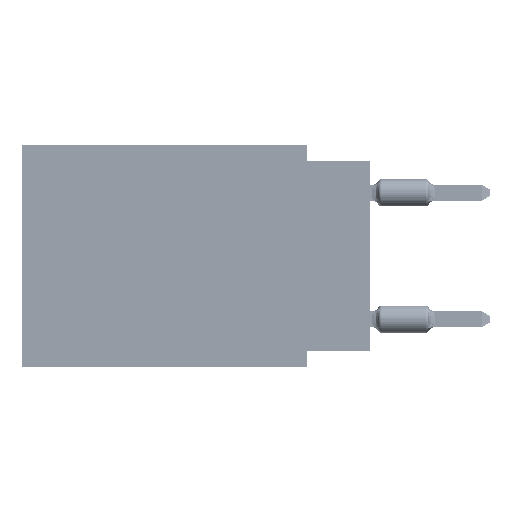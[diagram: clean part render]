
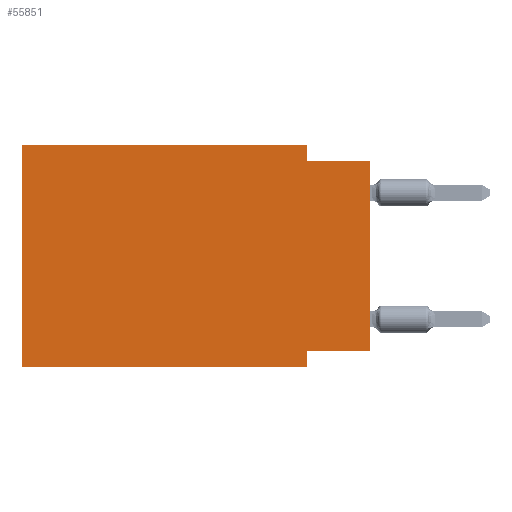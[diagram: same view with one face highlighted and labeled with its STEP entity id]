
A CAD part, left-side view. The second image highlights one B-rep face of the part: STEP entity #55851.
In plain terms, the highlighted planar face has unit normal (-1, 0, 0).
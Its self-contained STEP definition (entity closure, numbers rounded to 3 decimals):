
#151 = DIRECTION ( 'NONE',  ( 0., 0., 1. ) ) ;
#384 = CARTESIAN_POINT ( 'NONE',  ( 0., 2.54, -8.255 ) ) ;
#498 = LINE ( 'NONE', #28126, #64078 ) ;
#752 = LINE ( 'NONE', #40305, #62129 ) ;
#1316 = LINE ( 'NONE', #18832, #39171 ) ;
#3480 = EDGE_CURVE ( 'NONE', #56586, #4489, #69816, .T. ) ;
#4046 = FACE_OUTER_BOUND ( 'NONE', #61465, .T. ) ;
#4489 = VERTEX_POINT ( 'NONE', #43810 ) ;
#7274 = ORIENTED_EDGE ( 'NONE', *, *, #3480, .F. ) ;
#11560 = ORIENTED_EDGE ( 'NONE', *, *, #73206, .T. ) ;
#12030 = VERTEX_POINT ( 'NONE', #384 ) ;
#13238 = DIRECTION ( 'NONE',  ( 0., 0., 1. ) ) ;
#13810 = ORIENTED_EDGE ( 'NONE', *, *, #58039, .F. ) ;
#15136 = CARTESIAN_POINT ( 'NONE',  ( 0., 0., -0.635 ) ) ;
#16804 = VECTOR ( 'NONE', #53622, 1000. ) ;
#17238 = VERTEX_POINT ( 'NONE', #17566 ) ;
#17566 = CARTESIAN_POINT ( 'NONE',  ( 0., 2.54, -8.89 ) ) ;
#18680 = CARTESIAN_POINT ( 'NONE',  ( 0., 13.97, 0. ) ) ;
#18832 = CARTESIAN_POINT ( 'NONE',  ( 0., 0., 0. ) ) ;
#20469 = DIRECTION ( 'NONE',  ( 0., -1., 0. ) ) ;
#21967 = VECTOR ( 'NONE', #20469, 1000. ) ;
#23077 = DIRECTION ( 'NONE',  ( 0., 0., -1. ) ) ;
#25685 = CARTESIAN_POINT ( 'NONE',  ( 0., 13.97, -8.89 ) ) ;
#26681 = ORIENTED_EDGE ( 'NONE', *, *, #31737, .F. ) ;
#26885 = CARTESIAN_POINT ( 'NONE',  ( 0., 2.54, -0.635 ) ) ;
#28126 = CARTESIAN_POINT ( 'NONE',  ( 0., 0., -8.255 ) ) ;
#29567 = VECTOR ( 'NONE', #68330, 1000. ) ;
#31737 = EDGE_CURVE ( 'NONE', #34360, #44378, #38281, .T. ) ;
#34360 = VERTEX_POINT ( 'NONE', #26885 ) ;
#36318 = VERTEX_POINT ( 'NONE', #40016 ) ;
#38281 = LINE ( 'NONE', #67753, #40577 ) ;
#38374 = CARTESIAN_POINT ( 'NONE',  ( 0., 13.97, 0. ) ) ;
#39138 = ORIENTED_EDGE ( 'NONE', *, *, #44865, .F. ) ;
#39171 = VECTOR ( 'NONE', #13238, 1000. ) ;
#40016 = CARTESIAN_POINT ( 'NONE',  ( 0., 0., -8.255 ) ) ;
#40305 = CARTESIAN_POINT ( 'NONE',  ( 0., 2.54, -8.89 ) ) ;
#40577 = VECTOR ( 'NONE', #49110, 1000. ) ;
#40936 = LINE ( 'NONE', #41682, #16804 ) ;
#41682 = CARTESIAN_POINT ( 'NONE',  ( 0., 2.54, 0. ) ) ;
#43586 = AXIS2_PLACEMENT_3D ( 'NONE', #38374, #45809, #23077 ) ;
#43810 = CARTESIAN_POINT ( 'NONE',  ( 0., 2.54, 0. ) ) ;
#44072 = EDGE_CURVE ( 'NONE', #4489, #34360, #40936, .T. ) ;
#44378 = VERTEX_POINT ( 'NONE', #15136 ) ;
#44519 = LINE ( 'NONE', #67313, #54028 ) ;
#44865 = EDGE_CURVE ( 'NONE', #12030, #17238, #752, .T. ) ;
#45809 = DIRECTION ( 'NONE',  ( 1., 0., 0. ) ) ;
#46023 = ORIENTED_EDGE ( 'NONE', *, *, #49170, .T. ) ;
#46474 = CARTESIAN_POINT ( 'NONE',  ( 0., 13.97, -8.89 ) ) ;
#49031 = CARTESIAN_POINT ( 'NONE',  ( 0., 13.97, 0. ) ) ;
#49110 = DIRECTION ( 'NONE',  ( 0., -1., 0. ) ) ;
#49170 = EDGE_CURVE ( 'NONE', #56388, #17238, #60737, .T. ) ;
#53622 = DIRECTION ( 'NONE',  ( 0., 0., -1. ) ) ;
#54028 = VECTOR ( 'NONE', #151, 1000. ) ;
#55851 = ADVANCED_FACE ( 'NONE', ( #4046 ), #72357, .F. ) ;
#56388 = VERTEX_POINT ( 'NONE', #46474 ) ;
#56586 = VERTEX_POINT ( 'NONE', #49031 ) ;
#57839 = DIRECTION ( 'NONE',  ( 0., 0., -1. ) ) ;
#58039 = EDGE_CURVE ( 'NONE', #36318, #12030, #498, .T. ) ;
#60131 = ORIENTED_EDGE ( 'NONE', *, *, #44072, .F. ) ;
#60737 = LINE ( 'NONE', #25685, #21967 ) ;
#61465 = EDGE_LOOP ( 'NONE', ( #11560, #26681, #60131, #7274, #62051, #46023, #39138, #13810 ) ) ;
#62051 = ORIENTED_EDGE ( 'NONE', *, *, #68097, .F. ) ;
#62129 = VECTOR ( 'NONE', #57839, 1000. ) ;
#64078 = VECTOR ( 'NONE', #69527, 1000. ) ;
#67313 = CARTESIAN_POINT ( 'NONE',  ( 0., 13.97, 0. ) ) ;
#67753 = CARTESIAN_POINT ( 'NONE',  ( 0., 0., -0.635 ) ) ;
#68097 = EDGE_CURVE ( 'NONE', #56388, #56586, #44519, .T. ) ;
#68330 = DIRECTION ( 'NONE',  ( 0., -1., 0. ) ) ;
#69527 = DIRECTION ( 'NONE',  ( 0., 1., 0. ) ) ;
#69816 = LINE ( 'NONE', #18680, #29567 ) ;
#72357 = PLANE ( 'NONE',  #43586 ) ;
#73206 = EDGE_CURVE ( 'NONE', #36318, #44378, #1316, .T. ) ;
